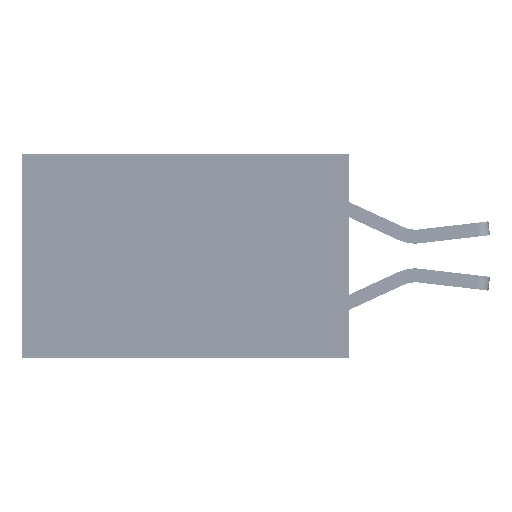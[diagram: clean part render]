
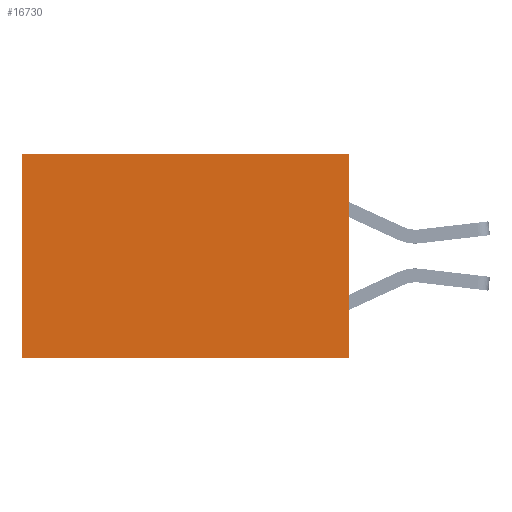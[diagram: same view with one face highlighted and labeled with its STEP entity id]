
A CAD part, left-side view. The second image highlights one B-rep face of the part: STEP entity #16730.
In plain terms, the highlighted planar face has unit normal (-1, 0, 0).
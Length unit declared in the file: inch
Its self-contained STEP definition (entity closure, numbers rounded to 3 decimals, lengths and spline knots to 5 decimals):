
#624 = ORIENTED_EDGE ( 'NONE', *, *, #8154, .F. ) ;
#2232 = DIRECTION ( 'NONE',  ( 0., 0., -1. ) ) ;
#2864 = ORIENTED_EDGE ( 'NONE', *, *, #20201, .F. ) ;
#3264 = ORIENTED_EDGE ( 'NONE', *, *, #20396, .T. ) ;
#5105 = LINE ( 'NONE', #11136, #30238 ) ;
#5946 = VECTOR ( 'NONE', #29845, 39.37008 ) ;
#8154 = EDGE_CURVE ( 'NONE', #29105, #9162, #17745, .T. ) ;
#8191 = DIRECTION ( 'NONE',  ( 0., 0., -1. ) ) ;
#9162 = VERTEX_POINT ( 'NONE', #11743 ) ;
#9899 = DIRECTION ( 'NONE',  ( 1., 0., 0. ) ) ;
#10945 = DIRECTION ( 'NONE',  ( 0., 0., -1. ) ) ;
#11069 = VECTOR ( 'NONE', #8191, 39.37008 ) ;
#11136 = CARTESIAN_POINT ( 'NONE',  ( 0.277, 0., -0.37 ) ) ;
#11302 = EDGE_LOOP ( 'NONE', ( #31810, #2864, #624, #3264 ) ) ;
#11330 = CARTESIAN_POINT ( 'NONE',  ( 0.277, 0.59, 0. ) ) ;
#11743 = CARTESIAN_POINT ( 'NONE',  ( 0.277, 0., -0.37 ) ) ;
#12352 = CARTESIAN_POINT ( 'NONE',  ( 0.277, 0., 0. ) ) ;
#13255 = AXIS2_PLACEMENT_3D ( 'NONE', #17449, #9899, #2232 ) ;
#13634 = VERTEX_POINT ( 'NONE', #11330 ) ;
#15823 = VECTOR ( 'NONE', #10945, 39.37008 ) ;
#16730 = ADVANCED_FACE ( 'NONE', ( #18601 ), #24883, .F. ) ;
#17037 = EDGE_CURVE ( 'NONE', #13634, #27866, #29131, .T. ) ;
#17449 = CARTESIAN_POINT ( 'NONE',  ( 0.277, 0., -0.37 ) ) ;
#17745 = LINE ( 'NONE', #18065, #11069 ) ;
#18065 = CARTESIAN_POINT ( 'NONE',  ( 0.277, 0., -0.37 ) ) ;
#18601 = FACE_OUTER_BOUND ( 'NONE', #11302, .T. ) ;
#20201 = EDGE_CURVE ( 'NONE', #9162, #27866, #5105, .T. ) ;
#20396 = EDGE_CURVE ( 'NONE', #29105, #13634, #31049, .T. ) ;
#20637 = CARTESIAN_POINT ( 'NONE',  ( 0.277, 0., 0. ) ) ;
#20935 = CARTESIAN_POINT ( 'NONE',  ( 0.277, 0.59, -0.37 ) ) ;
#21058 = CARTESIAN_POINT ( 'NONE',  ( 0.277, 0.59, -0.37 ) ) ;
#24883 = PLANE ( 'NONE',  #13255 ) ;
#26138 = DIRECTION ( 'NONE',  ( 0., 1., 0. ) ) ;
#27866 = VERTEX_POINT ( 'NONE', #21058 ) ;
#29105 = VERTEX_POINT ( 'NONE', #20637 ) ;
#29131 = LINE ( 'NONE', #20935, #15823 ) ;
#29845 = DIRECTION ( 'NONE',  ( 0., 1., 0. ) ) ;
#30238 = VECTOR ( 'NONE', #26138, 39.37008 ) ;
#31049 = LINE ( 'NONE', #12352, #5946 ) ;
#31810 = ORIENTED_EDGE ( 'NONE', *, *, #17037, .T. ) ;
